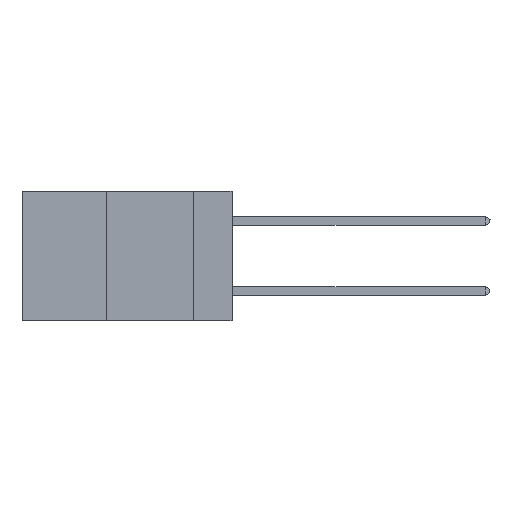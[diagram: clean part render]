
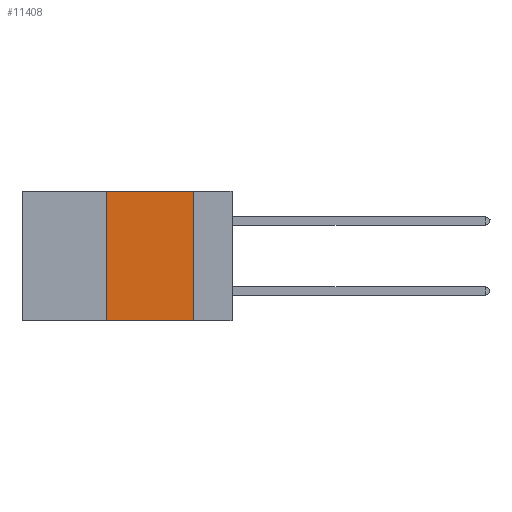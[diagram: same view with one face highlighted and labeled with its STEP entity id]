
A CAD part, left-side view. The second image highlights one B-rep face of the part: STEP entity #11408.
In plain terms, the highlighted planar face has unit normal (-1, 0, 0).
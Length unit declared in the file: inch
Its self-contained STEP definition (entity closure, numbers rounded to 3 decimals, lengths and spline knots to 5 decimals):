
#685 = DIRECTION ( 'NONE',  ( 0., 0., -1. ) ) ;
#1374 = VECTOR ( 'NONE', #14905, 39.37008 ) ;
#1738 = LINE ( 'NONE', #1887, #8923 ) ;
#1887 = CARTESIAN_POINT ( 'NONE',  ( 0., 0.6, 0. ) ) ;
#1936 = DIRECTION ( 'NONE',  ( 0., 0., -1. ) ) ;
#2176 = LINE ( 'NONE', #6845, #1374 ) ;
#2207 = ORIENTED_EDGE ( 'NONE', *, *, #6398, .T. ) ;
#3226 = CARTESIAN_POINT ( 'NONE',  ( 0., 0.11, 0. ) ) ;
#4200 = VERTEX_POINT ( 'NONE', #6598 ) ;
#4829 = ORIENTED_EDGE ( 'NONE', *, *, #7352, .F. ) ;
#5408 = CARTESIAN_POINT ( 'NONE',  ( 0., 0.6, -0.37 ) ) ;
#5800 = ORIENTED_EDGE ( 'NONE', *, *, #13236, .F. ) ;
#5953 = VECTOR ( 'NONE', #9933, 39.37008 ) ;
#6398 = EDGE_CURVE ( 'NONE', #11172, #11188, #14530, .T. ) ;
#6598 = CARTESIAN_POINT ( 'NONE',  ( 0., 0.11, 0. ) ) ;
#6845 = CARTESIAN_POINT ( 'NONE',  ( 0., 0.36, 0. ) ) ;
#7352 = EDGE_CURVE ( 'NONE', #4200, #11188, #8156, .T. ) ;
#7425 = VERTEX_POINT ( 'NONE', #13645 ) ;
#7646 = FACE_OUTER_BOUND ( 'NONE', #11282, .T. ) ;
#8156 = LINE ( 'NONE', #3226, #14646 ) ;
#8736 = ORIENTED_EDGE ( 'NONE', *, *, #11829, .F. ) ;
#8915 = AXIS2_PLACEMENT_3D ( 'NONE', #10160, #11162, #685 ) ;
#8923 = VECTOR ( 'NONE', #14439, 39.37008 ) ;
#9933 = DIRECTION ( 'NONE',  ( 0., -1., 0. ) ) ;
#10160 = CARTESIAN_POINT ( 'NONE',  ( 0., 0.6, 0. ) ) ;
#11162 = DIRECTION ( 'NONE',  ( 1., 0., 0. ) ) ;
#11172 = VERTEX_POINT ( 'NONE', #14232 ) ;
#11188 = VERTEX_POINT ( 'NONE', #11995 ) ;
#11282 = EDGE_LOOP ( 'NONE', ( #4829, #8736, #5800, #2207 ) ) ;
#11408 = ADVANCED_FACE ( 'NONE', ( #7646 ), #12306, .F. ) ;
#11829 = EDGE_CURVE ( 'NONE', #7425, #4200, #1738, .T. ) ;
#11995 = CARTESIAN_POINT ( 'NONE',  ( 0., 0.11, -0.37 ) ) ;
#12306 = PLANE ( 'NONE',  #8915 ) ;
#13236 = EDGE_CURVE ( 'NONE', #11172, #7425, #2176, .T. ) ;
#13645 = CARTESIAN_POINT ( 'NONE',  ( 0., 0.36, 0. ) ) ;
#14232 = CARTESIAN_POINT ( 'NONE',  ( 0., 0.36, -0.37 ) ) ;
#14439 = DIRECTION ( 'NONE',  ( 0., -1., 0. ) ) ;
#14530 = LINE ( 'NONE', #5408, #5953 ) ;
#14646 = VECTOR ( 'NONE', #1936, 39.37008 ) ;
#14905 = DIRECTION ( 'NONE',  ( 0., 0., 1. ) ) ;
